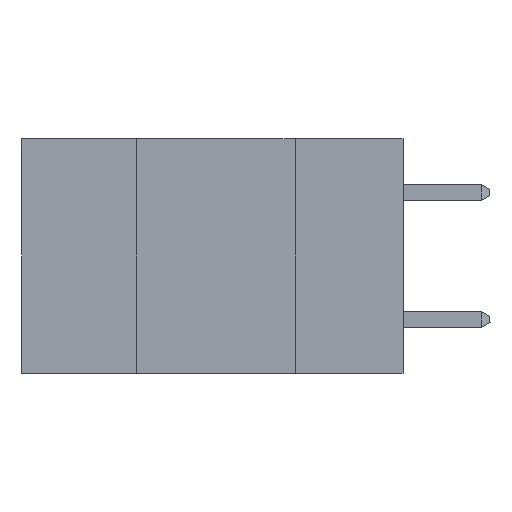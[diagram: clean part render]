
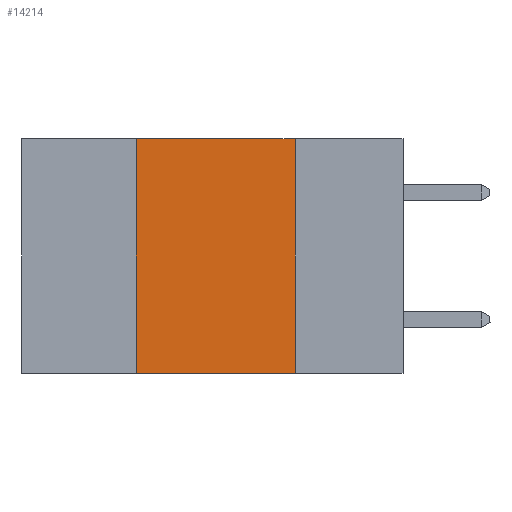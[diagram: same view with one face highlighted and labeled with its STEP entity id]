
A CAD part, left-side view. The second image highlights one B-rep face of the part: STEP entity #14214.
In plain terms, the highlighted planar face has unit normal (-1, 0, 0).
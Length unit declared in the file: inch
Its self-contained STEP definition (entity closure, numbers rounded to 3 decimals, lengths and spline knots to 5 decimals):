
#422 = ORIENTED_EDGE ( 'NONE', *, *, #6694, .F. ) ;
#608 = EDGE_LOOP ( 'NONE', ( #6813, #11163, #422, #4937 ) ) ;
#638 = CARTESIAN_POINT ( 'NONE',  ( 0., 0.42, 0. ) ) ;
#678 = DIRECTION ( 'NONE',  ( 0., 0., -1. ) ) ;
#1065 = DIRECTION ( 'NONE',  ( 1., 0., 0. ) ) ;
#1315 = VECTOR ( 'NONE', #19788, 39.37008 ) ;
#1852 = CARTESIAN_POINT ( 'NONE',  ( 0., 0.42, -0.37 ) ) ;
#2173 = VECTOR ( 'NONE', #13335, 39.37008 ) ;
#2483 = CARTESIAN_POINT ( 'NONE',  ( 0., 0.42, 0. ) ) ;
#2862 = CARTESIAN_POINT ( 'NONE',  ( 0., 0.6, 0. ) ) ;
#3132 = EDGE_CURVE ( 'NONE', #18558, #13116, #12201, .T. ) ;
#4937 = ORIENTED_EDGE ( 'NONE', *, *, #3132, .T. ) ;
#6694 = EDGE_CURVE ( 'NONE', #18558, #12680, #15229, .T. ) ;
#6813 = ORIENTED_EDGE ( 'NONE', *, *, #18091, .F. ) ;
#6852 = EDGE_CURVE ( 'NONE', #12680, #13723, #11466, .T. ) ;
#8474 = AXIS2_PLACEMENT_3D ( 'NONE', #16703, #1065, #13302 ) ;
#8732 = CARTESIAN_POINT ( 'NONE',  ( 0., 0.17, 0. ) ) ;
#11163 = ORIENTED_EDGE ( 'NONE', *, *, #6852, .F. ) ;
#11195 = FACE_OUTER_BOUND ( 'NONE', #608, .T. ) ;
#11466 = LINE ( 'NONE', #2862, #2173 ) ;
#11666 = VECTOR ( 'NONE', #17284, 39.37008 ) ;
#12201 = LINE ( 'NONE', #12627, #11666 ) ;
#12627 = CARTESIAN_POINT ( 'NONE',  ( 0., 0.6, -0.37 ) ) ;
#12680 = VERTEX_POINT ( 'NONE', #2483 ) ;
#12932 = CARTESIAN_POINT ( 'NONE',  ( 0., 0.17, 0. ) ) ;
#13116 = VERTEX_POINT ( 'NONE', #15742 ) ;
#13302 = DIRECTION ( 'NONE',  ( 0., 0., -1. ) ) ;
#13335 = DIRECTION ( 'NONE',  ( 0., -1., 0. ) ) ;
#13723 = VERTEX_POINT ( 'NONE', #8732 ) ;
#14214 = ADVANCED_FACE ( 'NONE', ( #11195 ), #21889, .F. ) ;
#15229 = LINE ( 'NONE', #638, #1315 ) ;
#15742 = CARTESIAN_POINT ( 'NONE',  ( 0., 0.17, -0.37 ) ) ;
#16703 = CARTESIAN_POINT ( 'NONE',  ( 0., 0.6, 0. ) ) ;
#17284 = DIRECTION ( 'NONE',  ( 0., -1., 0. ) ) ;
#18091 = EDGE_CURVE ( 'NONE', #13723, #13116, #20884, .T. ) ;
#18558 = VERTEX_POINT ( 'NONE', #1852 ) ;
#19788 = DIRECTION ( 'NONE',  ( 0., 0., 1. ) ) ;
#20355 = VECTOR ( 'NONE', #678, 39.37008 ) ;
#20884 = LINE ( 'NONE', #12932, #20355 ) ;
#21889 = PLANE ( 'NONE',  #8474 ) ;
